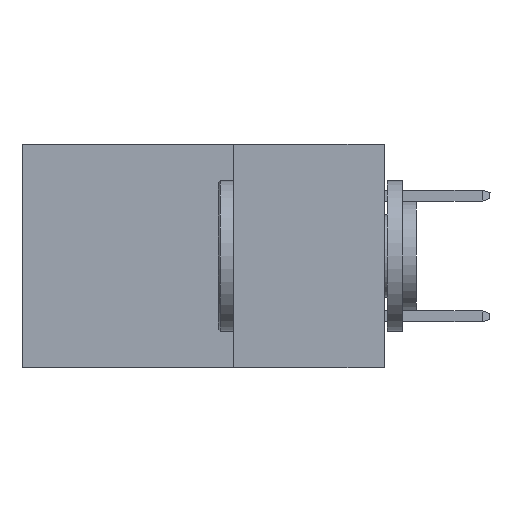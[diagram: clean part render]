
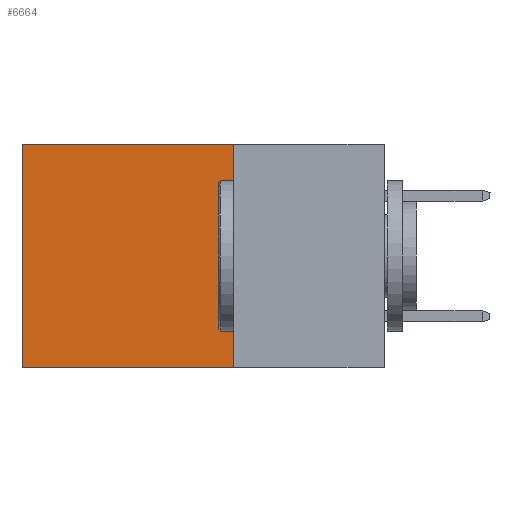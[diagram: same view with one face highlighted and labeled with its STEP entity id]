
A CAD part, left-side view. The second image highlights one B-rep face of the part: STEP entity #6664.
In plain terms, the highlighted planar face has unit normal (-1, 0, 0).
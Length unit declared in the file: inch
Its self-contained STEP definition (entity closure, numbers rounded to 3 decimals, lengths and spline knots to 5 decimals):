
#78 = LINE ( 'NONE', #9552, #5884 ) ;
#436 = AXIS2_PLACEMENT_3D ( 'NONE', #2172, #3157, #1449 ) ;
#545 = EDGE_LOOP ( 'NONE', ( #1416, #8161, #8049, #1342 ) ) ;
#1190 = PLANE ( 'NONE',  #436 ) ;
#1342 = ORIENTED_EDGE ( 'NONE', *, *, #6684, .T. ) ;
#1386 = CARTESIAN_POINT ( 'NONE',  ( 0.298, 0.25, 0. ) ) ;
#1416 = ORIENTED_EDGE ( 'NONE', *, *, #1856, .T. ) ;
#1449 = DIRECTION ( 'NONE',  ( 0., 0., -1. ) ) ;
#1856 = EDGE_CURVE ( 'NONE', #6987, #10568, #11828, .T. ) ;
#2172 = CARTESIAN_POINT ( 'NONE',  ( 0.298, 0.25, 0. ) ) ;
#3077 = VECTOR ( 'NONE', #7929, 39.37008 ) ;
#3157 = DIRECTION ( 'NONE',  ( 1., 0., 0. ) ) ;
#3391 = LINE ( 'NONE', #11807, #3077 ) ;
#4638 = EDGE_CURVE ( 'NONE', #5568, #10776, #3391, .T. ) ;
#4963 = VECTOR ( 'NONE', #12399, 39.37008 ) ;
#5568 = VERTEX_POINT ( 'NONE', #1386 ) ;
#5884 = VECTOR ( 'NONE', #9671, 39.37008 ) ;
#6323 = VECTOR ( 'NONE', #7375, 39.37008 ) ;
#6332 = EDGE_CURVE ( 'NONE', #10776, #10568, #78, .T. ) ;
#6664 = ADVANCED_FACE ( 'NONE', ( #11668 ), #1190, .F. ) ;
#6684 = EDGE_CURVE ( 'NONE', #5568, #6987, #9206, .T. ) ;
#6987 = VERTEX_POINT ( 'NONE', #10682 ) ;
#7219 = CARTESIAN_POINT ( 'NONE',  ( 0.298, 0.6, -0.37 ) ) ;
#7375 = DIRECTION ( 'NONE',  ( 0., 1., 0. ) ) ;
#7929 = DIRECTION ( 'NONE',  ( 0., 0., -1. ) ) ;
#8049 = ORIENTED_EDGE ( 'NONE', *, *, #4638, .F. ) ;
#8161 = ORIENTED_EDGE ( 'NONE', *, *, #6332, .F. ) ;
#9206 = LINE ( 'NONE', #9326, #6323 ) ;
#9326 = CARTESIAN_POINT ( 'NONE',  ( 0.298, 0.25, 0. ) ) ;
#9552 = CARTESIAN_POINT ( 'NONE',  ( 0.298, 0.25, -0.37 ) ) ;
#9671 = DIRECTION ( 'NONE',  ( 0., 1., 0. ) ) ;
#10568 = VERTEX_POINT ( 'NONE', #7219 ) ;
#10682 = CARTESIAN_POINT ( 'NONE',  ( 0.298, 0.6, 0. ) ) ;
#10776 = VERTEX_POINT ( 'NONE', #12625 ) ;
#11668 = FACE_OUTER_BOUND ( 'NONE', #545, .T. ) ;
#11807 = CARTESIAN_POINT ( 'NONE',  ( 0.298, 0.25, 0. ) ) ;
#11828 = LINE ( 'NONE', #12257, #4963 ) ;
#12257 = CARTESIAN_POINT ( 'NONE',  ( 0.298, 0.6, 0. ) ) ;
#12399 = DIRECTION ( 'NONE',  ( 0., 0., -1. ) ) ;
#12625 = CARTESIAN_POINT ( 'NONE',  ( 0.298, 0.25, -0.37 ) ) ;
